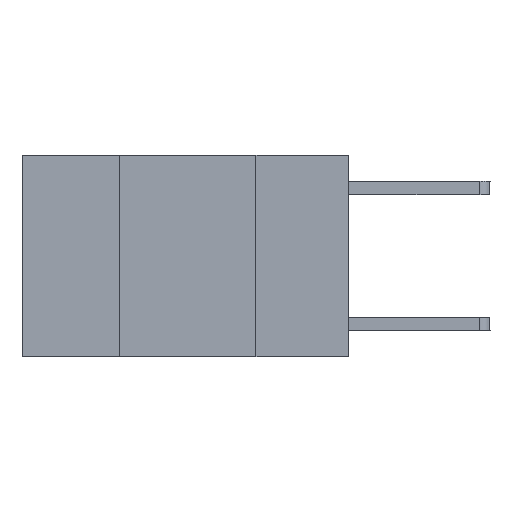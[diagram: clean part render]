
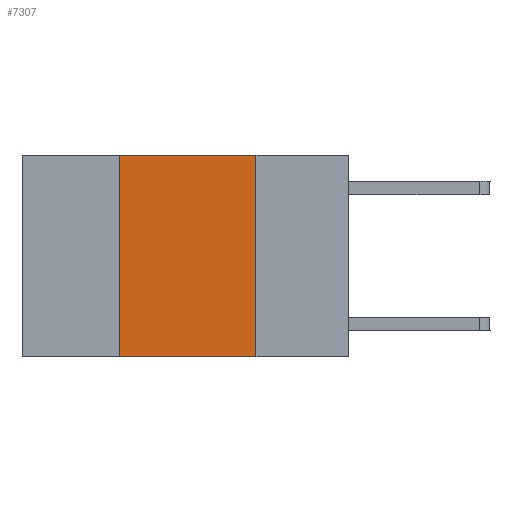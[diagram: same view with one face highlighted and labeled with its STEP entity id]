
A CAD part, left-side view. The second image highlights one B-rep face of the part: STEP entity #7307.
In plain terms, the highlighted planar face has unit normal (-1, 0, 0).
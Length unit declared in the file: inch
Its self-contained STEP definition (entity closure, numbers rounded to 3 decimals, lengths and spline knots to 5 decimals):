
#101 = DIRECTION ( 'NONE',  ( 1., 0., 0. ) ) ;
#674 = ORIENTED_EDGE ( 'NONE', *, *, #11873, .F. ) ;
#2035 = EDGE_CURVE ( 'NONE', #9996, #5003, #7489, .T. ) ;
#2866 = PLANE ( 'NONE',  #7927 ) ;
#3136 = EDGE_CURVE ( 'NONE', #5003, #9786, #9878, .T. ) ;
#4055 = ORIENTED_EDGE ( 'NONE', *, *, #10256, .T. ) ;
#5003 = VERTEX_POINT ( 'NONE', #10063 ) ;
#5015 = DIRECTION ( 'NONE',  ( 0., -1., 0. ) ) ;
#5909 = CARTESIAN_POINT ( 'NONE',  ( 0., 0.17, 0. ) ) ;
#6268 = DIRECTION ( 'NONE',  ( 0., 0., -1. ) ) ;
#6286 = DIRECTION ( 'NONE',  ( 0., 0., 1. ) ) ;
#6448 = VECTOR ( 'NONE', #6268, 39.37008 ) ;
#6969 = DIRECTION ( 'NONE',  ( 0., 0., -1. ) ) ;
#7211 = CARTESIAN_POINT ( 'NONE',  ( 0., 0.17, 0. ) ) ;
#7307 = ADVANCED_FACE ( 'NONE', ( #12568 ), #2866, .F. ) ;
#7489 = LINE ( 'NONE', #11133, #8016 ) ;
#7587 = ORIENTED_EDGE ( 'NONE', *, *, #2035, .F. ) ;
#7927 = AXIS2_PLACEMENT_3D ( 'NONE', #10669, #101, #6969 ) ;
#7999 = LINE ( 'NONE', #7211, #6448 ) ;
#8016 = VECTOR ( 'NONE', #6286, 39.37008 ) ;
#8306 = LINE ( 'NONE', #9534, #9680 ) ;
#8567 = DIRECTION ( 'NONE',  ( 0., -1., 0. ) ) ;
#8822 = CARTESIAN_POINT ( 'NONE',  ( 0., 0.42, -0.37 ) ) ;
#9250 = VERTEX_POINT ( 'NONE', #11338 ) ;
#9534 = CARTESIAN_POINT ( 'NONE',  ( 0., 0.6, -0.37 ) ) ;
#9680 = VECTOR ( 'NONE', #8567, 39.37008 ) ;
#9786 = VERTEX_POINT ( 'NONE', #5909 ) ;
#9878 = LINE ( 'NONE', #10841, #12296 ) ;
#9996 = VERTEX_POINT ( 'NONE', #8822 ) ;
#10063 = CARTESIAN_POINT ( 'NONE',  ( 0., 0.42, 0. ) ) ;
#10236 = ORIENTED_EDGE ( 'NONE', *, *, #3136, .F. ) ;
#10256 = EDGE_CURVE ( 'NONE', #9996, #9250, #8306, .T. ) ;
#10669 = CARTESIAN_POINT ( 'NONE',  ( 0., 0.6, 0. ) ) ;
#10841 = CARTESIAN_POINT ( 'NONE',  ( 0., 0.6, 0. ) ) ;
#11133 = CARTESIAN_POINT ( 'NONE',  ( 0., 0.42, 0. ) ) ;
#11338 = CARTESIAN_POINT ( 'NONE',  ( 0., 0.17, -0.37 ) ) ;
#11873 = EDGE_CURVE ( 'NONE', #9786, #9250, #7999, .T. ) ;
#12169 = EDGE_LOOP ( 'NONE', ( #674, #10236, #7587, #4055 ) ) ;
#12296 = VECTOR ( 'NONE', #5015, 39.37008 ) ;
#12568 = FACE_OUTER_BOUND ( 'NONE', #12169, .T. ) ;
